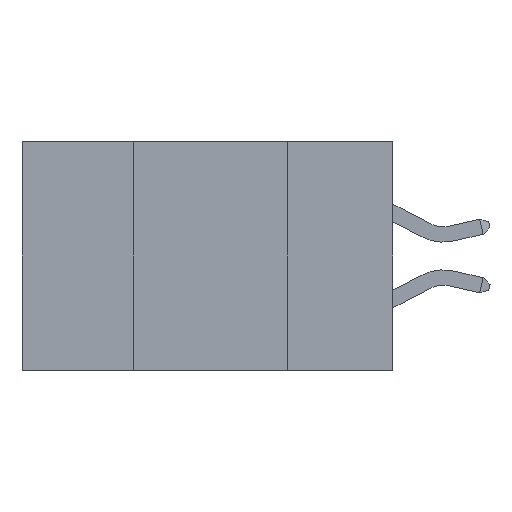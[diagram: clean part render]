
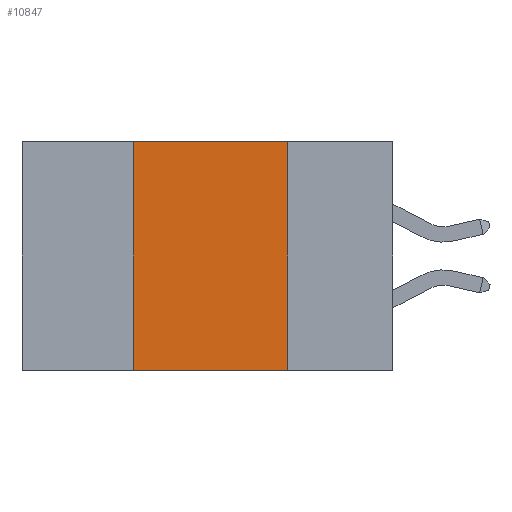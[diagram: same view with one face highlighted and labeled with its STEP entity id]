
A CAD part, left-side view. The second image highlights one B-rep face of the part: STEP entity #10847.
In plain terms, the highlighted planar face has unit normal (-1, 0, 0).
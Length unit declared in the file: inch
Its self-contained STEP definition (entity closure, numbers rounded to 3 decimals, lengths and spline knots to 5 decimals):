
#71 = DIRECTION ( 'NONE',  ( 0., 0., -1. ) ) ;
#545 = DIRECTION ( 'NONE',  ( 0., 0., -1. ) ) ;
#750 = EDGE_LOOP ( 'NONE', ( #24648, #7115, #15705, #7343 ) ) ;
#3551 = VECTOR ( 'NONE', #11455, 39.37008 ) ;
#4230 = LINE ( 'NONE', #22044, #3551 ) ;
#7000 = EDGE_CURVE ( 'NONE', #15844, #19937, #12634, .T. ) ;
#7115 = ORIENTED_EDGE ( 'NONE', *, *, #26975, .F. ) ;
#7199 = VERTEX_POINT ( 'NONE', #12646 ) ;
#7343 = ORIENTED_EDGE ( 'NONE', *, *, #7000, .T. ) ;
#7772 = DIRECTION ( 'NONE',  ( 0., -1., 0. ) ) ;
#9375 = CARTESIAN_POINT ( 'NONE',  ( 0., 0.6, 0. ) ) ;
#9423 = FACE_OUTER_BOUND ( 'NONE', #750, .T. ) ;
#10847 = ADVANCED_FACE ( 'NONE', ( #9423 ), #13496, .F. ) ;
#11455 = DIRECTION ( 'NONE',  ( 0., 0., 1. ) ) ;
#12634 = LINE ( 'NONE', #22335, #26240 ) ;
#12646 = CARTESIAN_POINT ( 'NONE',  ( 0., 0.42, 0. ) ) ;
#13496 = PLANE ( 'NONE',  #16631 ) ;
#14044 = VERTEX_POINT ( 'NONE', #18684 ) ;
#14336 = CARTESIAN_POINT ( 'NONE',  ( 0., 0.17, -0.37 ) ) ;
#15161 = CARTESIAN_POINT ( 'NONE',  ( 0., 0.17, 0. ) ) ;
#15705 = ORIENTED_EDGE ( 'NONE', *, *, #24818, .F. ) ;
#15844 = VERTEX_POINT ( 'NONE', #20872 ) ;
#16631 = AXIS2_PLACEMENT_3D ( 'NONE', #9375, #24149, #545 ) ;
#16653 = VECTOR ( 'NONE', #7772, 39.37008 ) ;
#18684 = CARTESIAN_POINT ( 'NONE',  ( 0., 0.17, 0. ) ) ;
#19937 = VERTEX_POINT ( 'NONE', #14336 ) ;
#20083 = EDGE_CURVE ( 'NONE', #14044, #19937, #26955, .T. ) ;
#20552 = DIRECTION ( 'NONE',  ( 0., -1., 0. ) ) ;
#20872 = CARTESIAN_POINT ( 'NONE',  ( 0., 0.42, -0.37 ) ) ;
#21972 = VECTOR ( 'NONE', #71, 39.37008 ) ;
#22044 = CARTESIAN_POINT ( 'NONE',  ( 0., 0.42, 0. ) ) ;
#22269 = LINE ( 'NONE', #26762, #16653 ) ;
#22335 = CARTESIAN_POINT ( 'NONE',  ( 0., 0.6, -0.37 ) ) ;
#24149 = DIRECTION ( 'NONE',  ( 1., 0., 0. ) ) ;
#24648 = ORIENTED_EDGE ( 'NONE', *, *, #20083, .F. ) ;
#24818 = EDGE_CURVE ( 'NONE', #15844, #7199, #4230, .T. ) ;
#26240 = VECTOR ( 'NONE', #20552, 39.37008 ) ;
#26762 = CARTESIAN_POINT ( 'NONE',  ( 0., 0.6, 0. ) ) ;
#26955 = LINE ( 'NONE', #15161, #21972 ) ;
#26975 = EDGE_CURVE ( 'NONE', #7199, #14044, #22269, .T. ) ;
